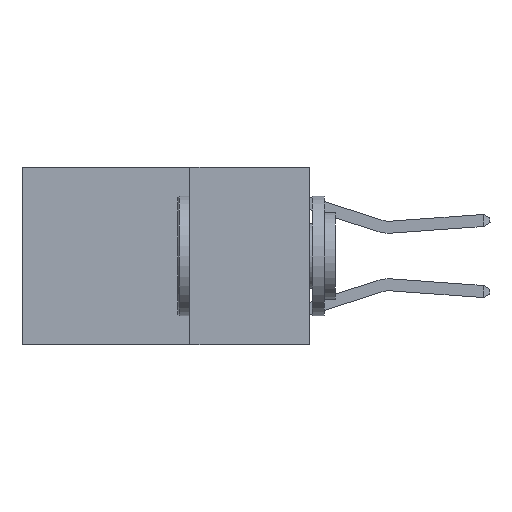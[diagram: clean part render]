
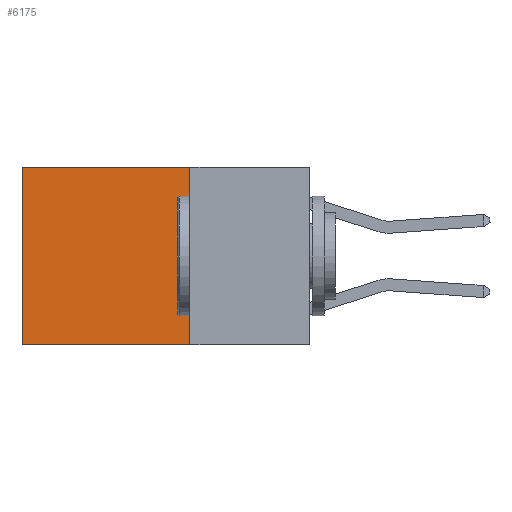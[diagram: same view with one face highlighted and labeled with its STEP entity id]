
A CAD part, left-side view. The second image highlights one B-rep face of the part: STEP entity #6175.
In plain terms, the highlighted planar face has unit normal (-1, 0, 0).
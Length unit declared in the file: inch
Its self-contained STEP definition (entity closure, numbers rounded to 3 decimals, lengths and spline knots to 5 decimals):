
#1076 = CARTESIAN_POINT ( 'NONE',  ( 0.2625, 0.25, 0. ) ) ;
#1173 = CARTESIAN_POINT ( 'NONE',  ( 0.2625, 0.25, -0.37 ) ) ;
#1185 = DIRECTION ( 'NONE',  ( 0., 1., 0. ) ) ;
#1248 = DIRECTION ( 'NONE',  ( 0., 1., 0. ) ) ;
#1261 = CARTESIAN_POINT ( 'NONE',  ( 0.2625, 0.25, 0. ) ) ;
#1743 = ORIENTED_EDGE ( 'NONE', *, *, #2425, .T. ) ;
#2133 = CARTESIAN_POINT ( 'NONE',  ( 0.2625, 0.6, 0. ) ) ;
#2425 = EDGE_CURVE ( 'NONE', #9245, #4191, #9665, .T. ) ;
#2426 = EDGE_CURVE ( 'NONE', #6665, #6761, #8131, .T. ) ;
#2807 = CARTESIAN_POINT ( 'NONE',  ( 0.2625, 0.25, -0.37 ) ) ;
#3925 = DIRECTION ( 'NONE',  ( 0., 0., -1. ) ) ;
#4191 = VERTEX_POINT ( 'NONE', #2133 ) ;
#4950 = LINE ( 'NONE', #6356, #7008 ) ;
#5492 = DIRECTION ( 'NONE',  ( 0., 0., -1. ) ) ;
#5594 = FACE_OUTER_BOUND ( 'NONE', #9787, .T. ) ;
#5716 = LINE ( 'NONE', #8837, #9531 ) ;
#6175 = ADVANCED_FACE ( 'NONE', ( #5594 ), #7776, .F. ) ;
#6241 = CARTESIAN_POINT ( 'NONE',  ( 0.2625, 0.25, 0. ) ) ;
#6356 = CARTESIAN_POINT ( 'NONE',  ( 0.2625, 0.6, 0. ) ) ;
#6665 = VERTEX_POINT ( 'NONE', #2807 ) ;
#6761 = VERTEX_POINT ( 'NONE', #9227 ) ;
#6875 = EDGE_CURVE ( 'NONE', #4191, #6761, #4950, .T. ) ;
#7008 = VECTOR ( 'NONE', #3925, 39.37008 ) ;
#7056 = EDGE_CURVE ( 'NONE', #9245, #6665, #5716, .T. ) ;
#7639 = VECTOR ( 'NONE', #1248, 39.37008 ) ;
#7776 = PLANE ( 'NONE',  #10218 ) ;
#7878 = VECTOR ( 'NONE', #1185, 39.37008 ) ;
#8131 = LINE ( 'NONE', #1173, #7878 ) ;
#8837 = CARTESIAN_POINT ( 'NONE',  ( 0.2625, 0.25, 0. ) ) ;
#8888 = ORIENTED_EDGE ( 'NONE', *, *, #6875, .T. ) ;
#9227 = CARTESIAN_POINT ( 'NONE',  ( 0.2625, 0.6, -0.37 ) ) ;
#9233 = ORIENTED_EDGE ( 'NONE', *, *, #7056, .F. ) ;
#9245 = VERTEX_POINT ( 'NONE', #1076 ) ;
#9304 = ORIENTED_EDGE ( 'NONE', *, *, #2426, .F. ) ;
#9531 = VECTOR ( 'NONE', #9578, 39.37008 ) ;
#9578 = DIRECTION ( 'NONE',  ( 0., 0., -1. ) ) ;
#9665 = LINE ( 'NONE', #1261, #7639 ) ;
#9787 = EDGE_LOOP ( 'NONE', ( #8888, #9304, #9233, #1743 ) ) ;
#10040 = DIRECTION ( 'NONE',  ( 1., 0., 0. ) ) ;
#10218 = AXIS2_PLACEMENT_3D ( 'NONE', #6241, #10040, #5492 ) ;
